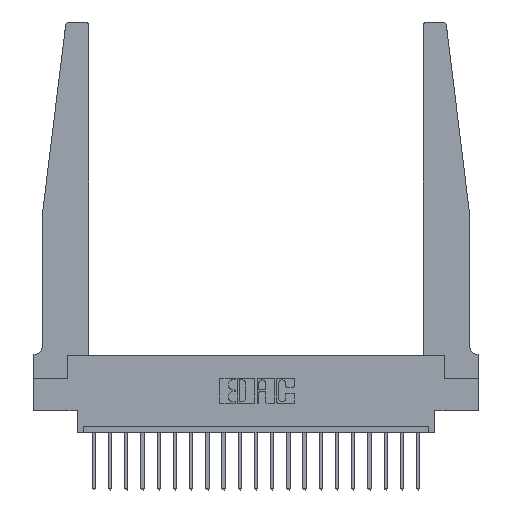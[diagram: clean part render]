
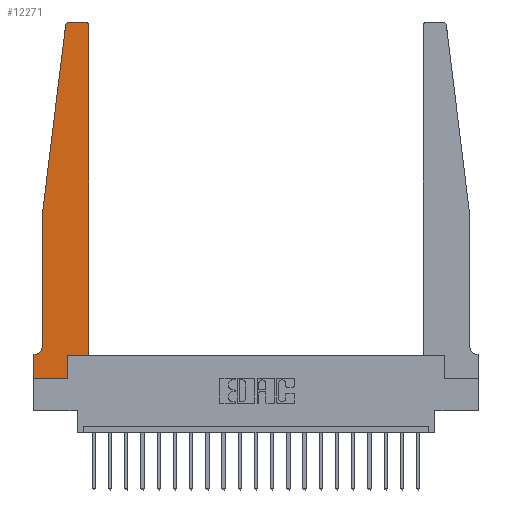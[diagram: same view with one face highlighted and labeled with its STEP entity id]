
A CAD part, top view. The second image highlights one B-rep face of the part: STEP entity #12271.
In plain terms, the highlighted planar face has unit normal (0, 0, 1).
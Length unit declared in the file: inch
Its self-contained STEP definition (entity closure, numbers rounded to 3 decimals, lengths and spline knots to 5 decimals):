
#38 = DIRECTION ( 'NONE',  ( -1., 0., 0. ) ) ;
#257 = EDGE_CURVE ( 'NONE', #388, #11689, #16350, .T. ) ;
#388 = VERTEX_POINT ( 'NONE', #7204 ) ;
#429 = LINE ( 'NONE', #15332, #8730 ) ;
#556 = CARTESIAN_POINT ( 'NONE',  ( 0., 0.1875, 0.37 ) ) ;
#712 = ORIENTED_EDGE ( 'NONE', *, *, #3021, .T. ) ;
#1175 = DIRECTION ( 'NONE',  ( 0., 0., 1. ) ) ;
#1181 = ORIENTED_EDGE ( 'NONE', *, *, #6631, .T. ) ;
#1276 = EDGE_CURVE ( 'NONE', #13136, #19775, #11077, .T. ) ;
#1324 = ORIENTED_EDGE ( 'NONE', *, *, #257, .T. ) ;
#1579 = VECTOR ( 'NONE', #6823, 39.37008 ) ;
#1640 = CARTESIAN_POINT ( 'NONE',  ( 0.25, 2.75, 0.37 ) ) ;
#1754 = CIRCLE ( 'NONE', #3459, 0.03 ) ;
#1850 = DIRECTION ( 'NONE',  ( 1., 0., 0. ) ) ;
#2231 = DIRECTION ( 'NONE',  ( -1., 0., 0. ) ) ;
#2404 = VERTEX_POINT ( 'NONE', #4632 ) ;
#2405 = VERTEX_POINT ( 'NONE', #7873 ) ;
#2579 = CARTESIAN_POINT ( 'NONE',  ( 0.395, 2.72, 0.37 ) ) ;
#2662 = DIRECTION ( 'NONE',  ( 0., 1., 0. ) ) ;
#3021 = EDGE_CURVE ( 'NONE', #19775, #16752, #429, .T. ) ;
#3137 = ORIENTED_EDGE ( 'NONE', *, *, #9094, .T. ) ;
#3459 = AXIS2_PLACEMENT_3D ( 'NONE', #2579, #12536, #12640 ) ;
#3526 = AXIS2_PLACEMENT_3D ( 'NONE', #16941, #4248, #2231 ) ;
#3571 = ORIENTED_EDGE ( 'NONE', *, *, #19691, .T. ) ;
#3843 = EDGE_CURVE ( 'NONE', #11689, #2404, #13535, .T. ) ;
#3861 = CIRCLE ( 'NONE', #3526, 0.05 ) ;
#3984 = ORIENTED_EDGE ( 'NONE', *, *, #14456, .T. ) ;
#4004 = LINE ( 'NONE', #11953, #8585 ) ;
#4051 = DIRECTION ( 'NONE',  ( 0., 1., 0. ) ) ;
#4142 = VECTOR ( 'NONE', #8906, 39.37008 ) ;
#4248 = DIRECTION ( 'NONE',  ( 0., 0., -1. ) ) ;
#4632 = CARTESIAN_POINT ( 'NONE',  ( 0.24675, 2.72367, 0.37 ) ) ;
#4793 = LINE ( 'NONE', #12534, #6254 ) ;
#5234 = ORIENTED_EDGE ( 'NONE', *, *, #10657, .T. ) ;
#5426 = LINE ( 'NONE', #13806, #14674 ) ;
#5561 = CARTESIAN_POINT ( 'NONE',  ( 0.2605, 0., 0.37 ) ) ;
#6254 = VECTOR ( 'NONE', #6404, 39.37008 ) ;
#6337 = VERTEX_POINT ( 'NONE', #7386 ) ;
#6404 = DIRECTION ( 'NONE',  ( 0., -1., 0. ) ) ;
#6538 = VERTEX_POINT ( 'NONE', #20037 ) ;
#6544 = CARTESIAN_POINT ( 'NONE',  ( 0.065, 0.2375, 0.37 ) ) ;
#6631 = EDGE_CURVE ( 'NONE', #6337, #2405, #14980, .T. ) ;
#6823 = DIRECTION ( 'NONE',  ( -1., 0., 0. ) ) ;
#7100 = DIRECTION ( 'NONE',  ( 0., 0., 1. ) ) ;
#7204 = CARTESIAN_POINT ( 'NONE',  ( 0.395, 2.75, 0.37 ) ) ;
#7386 = CARTESIAN_POINT ( 'NONE',  ( 0.015, 0.1875, 0.37 ) ) ;
#7716 = CARTESIAN_POINT ( 'NONE',  ( 0.27653, 2.72, 0.37 ) ) ;
#7873 = CARTESIAN_POINT ( 'NONE',  ( 0., 0.1875, 0.37 ) ) ;
#8306 = PLANE ( 'NONE',  #13161 ) ;
#8585 = VECTOR ( 'NONE', #10671, 39.37008 ) ;
#8691 = CARTESIAN_POINT ( 'NONE',  ( 0.425, 0.18, 0.37 ) ) ;
#8730 = VECTOR ( 'NONE', #4051, 39.37008 ) ;
#8782 = VERTEX_POINT ( 'NONE', #6544 ) ;
#8906 = DIRECTION ( 'NONE',  ( 1., 0., 0. ) ) ;
#9094 = EDGE_CURVE ( 'NONE', #14203, #8782, #4793, .T. ) ;
#9912 = ORIENTED_EDGE ( 'NONE', *, *, #19984, .T. ) ;
#10657 = EDGE_CURVE ( 'NONE', #8782, #6337, #3861, .T. ) ;
#10671 = DIRECTION ( 'NONE',  ( -0.122, -0.992, 0. ) ) ;
#11077 = LINE ( 'NONE', #20758, #16459 ) ;
#11136 = CARTESIAN_POINT ( 'NONE',  ( 0.065, 1.25, 0.37 ) ) ;
#11689 = VERTEX_POINT ( 'NONE', #19272 ) ;
#11828 = EDGE_LOOP ( 'NONE', ( #1324, #15517, #12279, #3137, #5234, #1181, #16573, #12015, #712, #3571, #3984, #9912 ) ) ;
#11953 = CARTESIAN_POINT ( 'NONE',  ( 0.065, 1.25, 0.37 ) ) ;
#12015 = ORIENTED_EDGE ( 'NONE', *, *, #1276, .T. ) ;
#12271 = ADVANCED_FACE ( 'NONE', ( #16774 ), #8306, .T. ) ;
#12279 = ORIENTED_EDGE ( 'NONE', *, *, #18844, .T. ) ;
#12534 = CARTESIAN_POINT ( 'NONE',  ( 0.065, 1.25, 0.37 ) ) ;
#12536 = DIRECTION ( 'NONE',  ( 0., 0., 1. ) ) ;
#12640 = DIRECTION ( 'NONE',  ( 1., 0., 0. ) ) ;
#12818 = CARTESIAN_POINT ( 'NONE',  ( 0.2605, 0.18, 0.37 ) ) ;
#13136 = VERTEX_POINT ( 'NONE', #19914 ) ;
#13161 = AXIS2_PLACEMENT_3D ( 'NONE', #556, #7100, #1850 ) ;
#13535 = CIRCLE ( 'NONE', #15964, 0.03 ) ;
#13608 = LINE ( 'NONE', #8691, #4142 ) ;
#13806 = CARTESIAN_POINT ( 'NONE',  ( 0.425, 0.18, 0.37 ) ) ;
#14203 = VERTEX_POINT ( 'NONE', #11136 ) ;
#14456 = EDGE_CURVE ( 'NONE', #6538, #20725, #5426, .T. ) ;
#14507 = EDGE_CURVE ( 'NONE', #2405, #13136, #18758, .T. ) ;
#14674 = VECTOR ( 'NONE', #2662, 39.37008 ) ;
#14980 = LINE ( 'NONE', #18421, #1579 ) ;
#15332 = CARTESIAN_POINT ( 'NONE',  ( 0.2605, 0.18, 0.37 ) ) ;
#15517 = ORIENTED_EDGE ( 'NONE', *, *, #3843, .T. ) ;
#15700 = VECTOR ( 'NONE', #38, 39.37008 ) ;
#15964 = AXIS2_PLACEMENT_3D ( 'NONE', #7716, #1175, #16087 ) ;
#16087 = DIRECTION ( 'NONE',  ( 1., 0., 0. ) ) ;
#16350 = LINE ( 'NONE', #1640, #15700 ) ;
#16459 = VECTOR ( 'NONE', #17621, 39.37008 ) ;
#16573 = ORIENTED_EDGE ( 'NONE', *, *, #14507, .T. ) ;
#16752 = VERTEX_POINT ( 'NONE', #12818 ) ;
#16774 = FACE_OUTER_BOUND ( 'NONE', #11828, .T. ) ;
#16941 = CARTESIAN_POINT ( 'NONE',  ( 0.015, 0.2375, 0.37 ) ) ;
#17145 = DIRECTION ( 'NONE',  ( 0., -1., 0. ) ) ;
#17621 = DIRECTION ( 'NONE',  ( 1., 0., 0. ) ) ;
#18421 = CARTESIAN_POINT ( 'NONE',  ( 0.065, 0.1875, 0.37 ) ) ;
#18758 = LINE ( 'NONE', #18863, #19823 ) ;
#18844 = EDGE_CURVE ( 'NONE', #2404, #14203, #4004, .T. ) ;
#18863 = CARTESIAN_POINT ( 'NONE',  ( 0., 0., 0.37 ) ) ;
#19272 = CARTESIAN_POINT ( 'NONE',  ( 0.27653, 2.75, 0.37 ) ) ;
#19691 = EDGE_CURVE ( 'NONE', #16752, #6538, #13608, .T. ) ;
#19775 = VERTEX_POINT ( 'NONE', #5561 ) ;
#19823 = VECTOR ( 'NONE', #17145, 39.37008 ) ;
#19914 = CARTESIAN_POINT ( 'NONE',  ( 0., 0., 0.37 ) ) ;
#19984 = EDGE_CURVE ( 'NONE', #20725, #388, #1754, .T. ) ;
#20037 = CARTESIAN_POINT ( 'NONE',  ( 0.425, 0.18, 0.37 ) ) ;
#20725 = VERTEX_POINT ( 'NONE', #21055 ) ;
#20758 = CARTESIAN_POINT ( 'NONE',  ( 0., 0., 0.37 ) ) ;
#21055 = CARTESIAN_POINT ( 'NONE',  ( 0.425, 2.72, 0.37 ) ) ;
